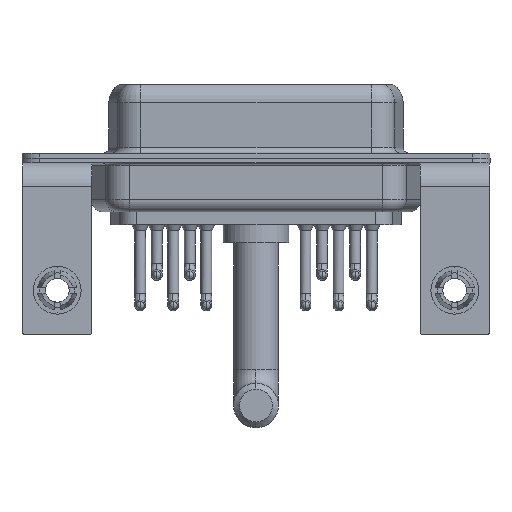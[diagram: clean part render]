
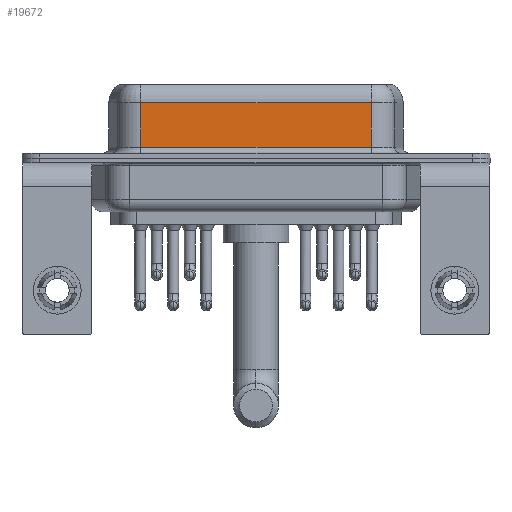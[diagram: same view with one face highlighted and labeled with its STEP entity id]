
A CAD part, front view. The second image highlights one B-rep face of the part: STEP entity #19672.
In plain terms, the highlighted planar face has unit normal (0, -1, 0).
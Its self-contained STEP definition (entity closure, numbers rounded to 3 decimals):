
#1148 = VERTEX_POINT ( 'NONE', #19311 ) ;
#1432 = DIRECTION ( 'NONE',  ( 0., 1., 0. ) ) ;
#1909 = EDGE_CURVE ( 'NONE', #1148, #17974, #20636, .T. ) ;
#1916 = CARTESIAN_POINT ( 'NONE',  ( 26.287, -3.95, 0.9 ) ) ;
#2299 = CARTESIAN_POINT ( 'NONE',  ( 7.013, -3.95, 6.4 ) ) ;
#2792 = EDGE_CURVE ( 'NONE', #17974, #19152, #3896, .T. ) ;
#3896 = LINE ( 'NONE', #2299, #19661 ) ;
#4173 = VERTEX_POINT ( 'NONE', #17932 ) ;
#6493 = LINE ( 'NONE', #1916, #8456 ) ;
#7378 = EDGE_CURVE ( 'NONE', #1148, #4173, #11604, .T. ) ;
#7866 = EDGE_LOOP ( 'NONE', ( #16099, #20330, #20727, #19627 ) ) ;
#7997 = DIRECTION ( 'NONE',  ( 0., 0., -1. ) ) ;
#8354 = CARTESIAN_POINT ( 'NONE',  ( 7.013, -3.95, 4.65 ) ) ;
#8456 = VECTOR ( 'NONE', #16508, 1000. ) ;
#9109 = PLANE ( 'NONE',  #14285 ) ;
#10116 = CARTESIAN_POINT ( 'NONE',  ( 7.013, -3.95, 0.9 ) ) ;
#11015 = CARTESIAN_POINT ( 'NONE',  ( 26.287, -3.95, 6.4 ) ) ;
#11047 = VECTOR ( 'NONE', #12826, 1000. ) ;
#11604 = LINE ( 'NONE', #13202, #16108 ) ;
#12826 = DIRECTION ( 'NONE',  ( -1., 0., 0. ) ) ;
#13202 = CARTESIAN_POINT ( 'NONE',  ( 26.287, -3.95, 6.4 ) ) ;
#14285 = AXIS2_PLACEMENT_3D ( 'NONE', #11015, #1432, #15815 ) ;
#15815 = DIRECTION ( 'NONE',  ( 0., 0., 1. ) ) ;
#16025 = FACE_OUTER_BOUND ( 'NONE', #7866, .T. ) ;
#16099 = ORIENTED_EDGE ( 'NONE', *, *, #7378, .F. ) ;
#16108 = VECTOR ( 'NONE', #7997, 1000. ) ;
#16508 = DIRECTION ( 'NONE',  ( 1., 0., 0. ) ) ;
#17932 = CARTESIAN_POINT ( 'NONE',  ( 26.287, -3.95, 0.9 ) ) ;
#17974 = VERTEX_POINT ( 'NONE', #8354 ) ;
#19095 = EDGE_CURVE ( 'NONE', #19152, #4173, #6493, .T. ) ;
#19152 = VERTEX_POINT ( 'NONE', #10116 ) ;
#19311 = CARTESIAN_POINT ( 'NONE',  ( 26.287, -3.95, 4.65 ) ) ;
#19456 = CARTESIAN_POINT ( 'NONE',  ( 26.287, -3.95, 4.65 ) ) ;
#19627 = ORIENTED_EDGE ( 'NONE', *, *, #19095, .T. ) ;
#19661 = VECTOR ( 'NONE', #20113, 1000. ) ;
#19672 = ADVANCED_FACE ( 'NONE', ( #16025 ), #9109, .F. ) ;
#20113 = DIRECTION ( 'NONE',  ( 0., 0., -1. ) ) ;
#20330 = ORIENTED_EDGE ( 'NONE', *, *, #1909, .T. ) ;
#20636 = LINE ( 'NONE', #19456, #11047 ) ;
#20727 = ORIENTED_EDGE ( 'NONE', *, *, #2792, .T. ) ;
